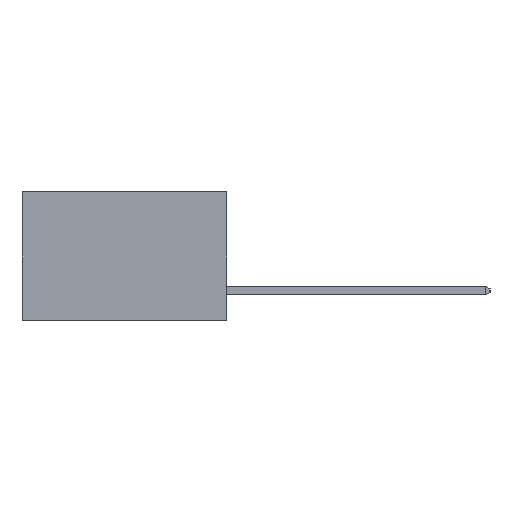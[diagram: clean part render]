
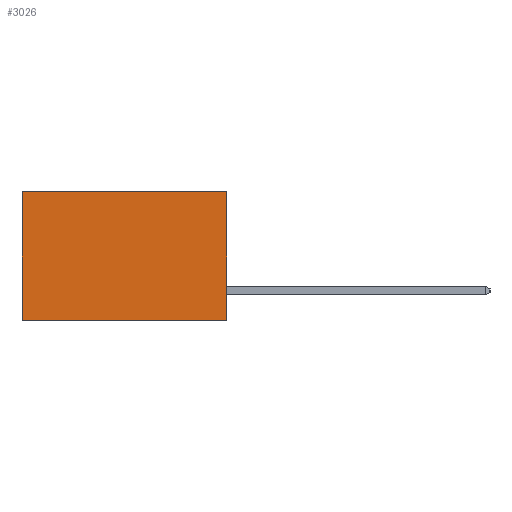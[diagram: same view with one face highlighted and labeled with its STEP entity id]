
A CAD part, left-side view. The second image highlights one B-rep face of the part: STEP entity #3026.
In plain terms, the highlighted planar face has unit normal (-1, 0, 0).
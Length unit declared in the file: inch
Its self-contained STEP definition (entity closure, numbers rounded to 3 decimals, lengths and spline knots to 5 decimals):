
#243 = DIRECTION ( 'NONE',  ( 0., 1., 0. ) ) ;
#318 = CARTESIAN_POINT ( 'NONE',  ( 0.277, 0., 0. ) ) ;
#1175 = CARTESIAN_POINT ( 'NONE',  ( 0.277, 0., -0.37 ) ) ;
#1373 = LINE ( 'NONE', #20781, #14322 ) ;
#1438 = DIRECTION ( 'NONE',  ( 0., 0., -1. ) ) ;
#1497 = FACE_OUTER_BOUND ( 'NONE', #10518, .T. ) ;
#2200 = EDGE_CURVE ( 'NONE', #15516, #13608, #9710, .T. ) ;
#2774 = CARTESIAN_POINT ( 'NONE',  ( 0.277, 0.59, 0. ) ) ;
#3026 = ADVANCED_FACE ( 'NONE', ( #1497 ), #11334, .F. ) ;
#7666 = EDGE_CURVE ( 'NONE', #13619, #11001, #9007, .T. ) ;
#8403 = AXIS2_PLACEMENT_3D ( 'NONE', #12768, #11315, #11454 ) ;
#8483 = VECTOR ( 'NONE', #10604, 39.37008 ) ;
#9007 = LINE ( 'NONE', #10599, #8483 ) ;
#9142 = DIRECTION ( 'NONE',  ( 0., 0., -1. ) ) ;
#9152 = ORIENTED_EDGE ( 'NONE', *, *, #2200, .T. ) ;
#9196 = VECTOR ( 'NONE', #243, 39.37008 ) ;
#9710 = LINE ( 'NONE', #318, #9196 ) ;
#10518 = EDGE_LOOP ( 'NONE', ( #12610, #11522, #16907, #9152 ) ) ;
#10599 = CARTESIAN_POINT ( 'NONE',  ( 0.277, 0., -0.37 ) ) ;
#10604 = DIRECTION ( 'NONE',  ( 0., 1., 0. ) ) ;
#11001 = VERTEX_POINT ( 'NONE', #20826 ) ;
#11315 = DIRECTION ( 'NONE',  ( 1., 0., 0. ) ) ;
#11334 = PLANE ( 'NONE',  #8403 ) ;
#11454 = DIRECTION ( 'NONE',  ( 0., 0., -1. ) ) ;
#11522 = ORIENTED_EDGE ( 'NONE', *, *, #7666, .F. ) ;
#12610 = ORIENTED_EDGE ( 'NONE', *, *, #15727, .T. ) ;
#12768 = CARTESIAN_POINT ( 'NONE',  ( 0.277, 0., -0.37 ) ) ;
#13466 = LINE ( 'NONE', #17147, #16221 ) ;
#13608 = VERTEX_POINT ( 'NONE', #2774 ) ;
#13619 = VERTEX_POINT ( 'NONE', #1175 ) ;
#14322 = VECTOR ( 'NONE', #1438, 39.37008 ) ;
#15516 = VERTEX_POINT ( 'NONE', #16661 ) ;
#15727 = EDGE_CURVE ( 'NONE', #13608, #11001, #13466, .T. ) ;
#16221 = VECTOR ( 'NONE', #9142, 39.37008 ) ;
#16661 = CARTESIAN_POINT ( 'NONE',  ( 0.277, 0., 0. ) ) ;
#16907 = ORIENTED_EDGE ( 'NONE', *, *, #18664, .F. ) ;
#17147 = CARTESIAN_POINT ( 'NONE',  ( 0.277, 0.59, -0.37 ) ) ;
#18664 = EDGE_CURVE ( 'NONE', #15516, #13619, #1373, .T. ) ;
#20781 = CARTESIAN_POINT ( 'NONE',  ( 0.277, 0., -0.37 ) ) ;
#20826 = CARTESIAN_POINT ( 'NONE',  ( 0.277, 0.59, -0.37 ) ) ;
